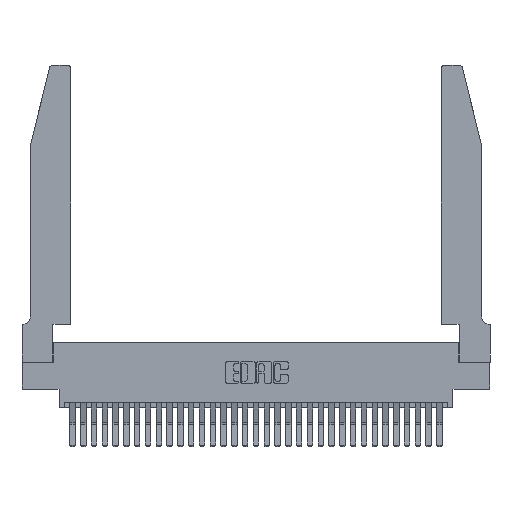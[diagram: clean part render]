
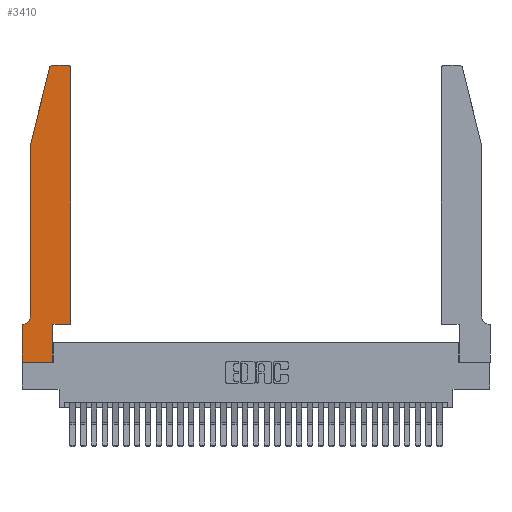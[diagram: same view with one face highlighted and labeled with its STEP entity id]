
A CAD part, top view. The second image highlights one B-rep face of the part: STEP entity #3410.
In plain terms, the highlighted planar face has unit normal (0, 0, 1).
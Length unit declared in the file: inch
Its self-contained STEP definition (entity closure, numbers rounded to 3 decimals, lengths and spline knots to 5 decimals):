
#9 = VERTEX_POINT ( 'NONE', #6645 ) ;
#365 = EDGE_CURVE ( 'NONE', #8291, #15857, #28043, .T. ) ;
#1519 = ORIENTED_EDGE ( 'NONE', *, *, #9588, .T. ) ;
#1732 = CARTESIAN_POINT ( 'NONE',  ( 0.4205, 2.75, 0.37 ) ) ;
#1916 = ORIENTED_EDGE ( 'NONE', *, *, #3328, .T. ) ;
#1991 = EDGE_CURVE ( 'NONE', #15857, #21906, #31522, .T. ) ;
#2311 = AXIS2_PLACEMENT_3D ( 'NONE', #21824, #6220, #29677 ) ;
#2326 = VERTEX_POINT ( 'NONE', #11396 ) ;
#2431 = EDGE_LOOP ( 'NONE', ( #30378, #1519, #8329, #24557, #3120, #1916, #24049, #24135, #22053, #6563, #23705, #18529 ) ) ;
#3025 = CARTESIAN_POINT ( 'NONE',  ( 0.284, 2.72, 0.37 ) ) ;
#3120 = ORIENTED_EDGE ( 'NONE', *, *, #19485, .T. ) ;
#3127 = VECTOR ( 'NONE', #28720, 39.37008 ) ;
#3328 = EDGE_CURVE ( 'NONE', #9, #9495, #19966, .T. ) ;
#3410 = ADVANCED_FACE ( 'NONE', ( #30865 ), #9751, .T. ) ;
#3849 = LINE ( 'NONE', #7949, #15952 ) ;
#3889 = VERTEX_POINT ( 'NONE', #4522 ) ;
#4253 = DIRECTION ( 'NONE',  ( 0., 0., -1. ) ) ;
#4449 = DIRECTION ( 'NONE',  ( -1., 0., 0. ) ) ;
#4522 = CARTESIAN_POINT ( 'NONE',  ( 0.2865, 0.35, 0.37 ) ) ;
#5129 = CARTESIAN_POINT ( 'NONE',  ( 0., 0., 0.37 ) ) ;
#5271 = DIRECTION ( 'NONE',  ( 1., 0., 0. ) ) ;
#5591 = CIRCLE ( 'NONE', #26213, 0.03 ) ;
#5623 = EDGE_CURVE ( 'NONE', #9495, #16169, #15741, .T. ) ;
#6220 = DIRECTION ( 'NONE',  ( 0., 0., 1. ) ) ;
#6333 = CARTESIAN_POINT ( 'NONE',  ( 0.25487, 2.72718, 0.37 ) ) ;
#6533 = CARTESIAN_POINT ( 'NONE',  ( 0.4505, 2.72, 0.37 ) ) ;
#6563 = ORIENTED_EDGE ( 'NONE', *, *, #8930, .T. ) ;
#6645 = CARTESIAN_POINT ( 'NONE',  ( 0.0055, 0.35, 0.37 ) ) ;
#6795 = CARTESIAN_POINT ( 'NONE',  ( 0.4505, 0.35, 0.37 ) ) ;
#7836 = DIRECTION ( 'NONE',  ( 0., 1., 0. ) ) ;
#7949 = CARTESIAN_POINT ( 'NONE',  ( 0.2865, 0.35, 0.37 ) ) ;
#8047 = CARTESIAN_POINT ( 'NONE',  ( 0.2605, 2.75, 0.37 ) ) ;
#8051 = VECTOR ( 'NONE', #25863, 39.37008 ) ;
#8291 = VERTEX_POINT ( 'NONE', #32080 ) ;
#8329 = ORIENTED_EDGE ( 'NONE', *, *, #17070, .T. ) ;
#8495 = CARTESIAN_POINT ( 'NONE',  ( 0., 0.35, 0.37 ) ) ;
#8771 = CARTESIAN_POINT ( 'NONE',  ( 0.2865, 0., 0.37 ) ) ;
#8930 = EDGE_CURVE ( 'NONE', #3889, #8291, #25264, .T. ) ;
#9201 = DIRECTION ( 'NONE',  ( -0.239, -0.971, 0. ) ) ;
#9495 = VERTEX_POINT ( 'NONE', #8495 ) ;
#9588 = EDGE_CURVE ( 'NONE', #21688, #11720, #5591, .T. ) ;
#9751 = PLANE ( 'NONE',  #31326 ) ;
#9816 = VECTOR ( 'NONE', #11977, 39.37008 ) ;
#10732 = VECTOR ( 'NONE', #23227, 39.37008 ) ;
#10814 = LINE ( 'NONE', #8047, #3127 ) ;
#10822 = DIRECTION ( 'NONE',  ( 0., 0., 1. ) ) ;
#11381 = VERTEX_POINT ( 'NONE', #8771 ) ;
#11396 = CARTESIAN_POINT ( 'NONE',  ( 0.0755, 2., 0.37 ) ) ;
#11720 = VERTEX_POINT ( 'NONE', #6333 ) ;
#11926 = VECTOR ( 'NONE', #4449, 39.37008 ) ;
#11977 = DIRECTION ( 'NONE',  ( 0., -1., 0. ) ) ;
#12234 = CARTESIAN_POINT ( 'NONE',  ( 0., 0.35, 0.37 ) ) ;
#12262 = CIRCLE ( 'NONE', #17901, 0.07 ) ;
#12445 = DIRECTION ( 'NONE',  ( 0., 0., 1. ) ) ;
#13441 = CARTESIAN_POINT ( 'NONE',  ( 0., 0., 0.37 ) ) ;
#13481 = EDGE_CURVE ( 'NONE', #2326, #32595, #22716, .T. ) ;
#14520 = CARTESIAN_POINT ( 'NONE',  ( 0.0055, 0.42, 0.37 ) ) ;
#15737 = CARTESIAN_POINT ( 'NONE',  ( 0.0755, 2., 0.37 ) ) ;
#15741 = LINE ( 'NONE', #5129, #8051 ) ;
#15857 = VERTEX_POINT ( 'NONE', #6533 ) ;
#15871 = EDGE_CURVE ( 'NONE', #16169, #11381, #29755, .T. ) ;
#15952 = VECTOR ( 'NONE', #7836, 39.37008 ) ;
#16169 = VERTEX_POINT ( 'NONE', #13441 ) ;
#17039 = EDGE_CURVE ( 'NONE', #21906, #21688, #10814, .T. ) ;
#17070 = EDGE_CURVE ( 'NONE', #11720, #2326, #20068, .T. ) ;
#17901 = AXIS2_PLACEMENT_3D ( 'NONE', #14520, #4253, #22040 ) ;
#18529 = ORIENTED_EDGE ( 'NONE', *, *, #1991, .T. ) ;
#19485 = EDGE_CURVE ( 'NONE', #32595, #9, #12262, .T. ) ;
#19738 = CARTESIAN_POINT ( 'NONE',  ( 0.0755, 0.42, 0.37 ) ) ;
#19966 = LINE ( 'NONE', #28030, #11926 ) ;
#20068 = LINE ( 'NONE', #15737, #30203 ) ;
#21688 = VERTEX_POINT ( 'NONE', #24777 ) ;
#21824 = CARTESIAN_POINT ( 'NONE',  ( 0.4205, 2.72, 0.37 ) ) ;
#21906 = VERTEX_POINT ( 'NONE', #1732 ) ;
#22040 = DIRECTION ( 'NONE',  ( -1., 0., 0. ) ) ;
#22053 = ORIENTED_EDGE ( 'NONE', *, *, #27771, .T. ) ;
#22716 = LINE ( 'NONE', #27430, #9816 ) ;
#23227 = DIRECTION ( 'NONE',  ( 1., 0., 0. ) ) ;
#23705 = ORIENTED_EDGE ( 'NONE', *, *, #365, .T. ) ;
#24049 = ORIENTED_EDGE ( 'NONE', *, *, #5623, .T. ) ;
#24135 = ORIENTED_EDGE ( 'NONE', *, *, #15871, .T. ) ;
#24557 = ORIENTED_EDGE ( 'NONE', *, *, #13481, .T. ) ;
#24587 = DIRECTION ( 'NONE',  ( 0., 1., 0. ) ) ;
#24777 = CARTESIAN_POINT ( 'NONE',  ( 0.284, 2.75, 0.37 ) ) ;
#25264 = LINE ( 'NONE', #29983, #32124 ) ;
#25863 = DIRECTION ( 'NONE',  ( 0., -1., 0. ) ) ;
#26213 = AXIS2_PLACEMENT_3D ( 'NONE', #3025, #10822, #31043 ) ;
#27168 = CARTESIAN_POINT ( 'NONE',  ( 0., 0., 0.37 ) ) ;
#27430 = CARTESIAN_POINT ( 'NONE',  ( 0.0755, 2., 0.37 ) ) ;
#27771 = EDGE_CURVE ( 'NONE', #11381, #3889, #3849, .T. ) ;
#28030 = CARTESIAN_POINT ( 'NONE',  ( 0.0755, 0.35, 0.37 ) ) ;
#28043 = LINE ( 'NONE', #6795, #29649 ) ;
#28140 = DIRECTION ( 'NONE',  ( 1., 0., 0. ) ) ;
#28720 = DIRECTION ( 'NONE',  ( -1., 0., 0. ) ) ;
#29649 = VECTOR ( 'NONE', #24587, 39.37008 ) ;
#29677 = DIRECTION ( 'NONE',  ( 1., 0., 0. ) ) ;
#29755 = LINE ( 'NONE', #27168, #10732 ) ;
#29983 = CARTESIAN_POINT ( 'NONE',  ( 0.4505, 0.35, 0.37 ) ) ;
#30203 = VECTOR ( 'NONE', #9201, 39.37008 ) ;
#30378 = ORIENTED_EDGE ( 'NONE', *, *, #17039, .T. ) ;
#30865 = FACE_OUTER_BOUND ( 'NONE', #2431, .T. ) ;
#31043 = DIRECTION ( 'NONE',  ( 1., 0., 0. ) ) ;
#31326 = AXIS2_PLACEMENT_3D ( 'NONE', #12234, #12445, #28140 ) ;
#31522 = CIRCLE ( 'NONE', #2311, 0.03 ) ;
#32080 = CARTESIAN_POINT ( 'NONE',  ( 0.4505, 0.35, 0.37 ) ) ;
#32124 = VECTOR ( 'NONE', #5271, 39.37008 ) ;
#32595 = VERTEX_POINT ( 'NONE', #19738 ) ;
